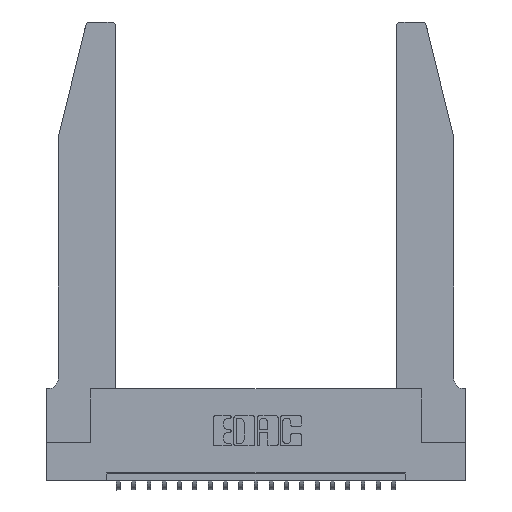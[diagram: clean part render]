
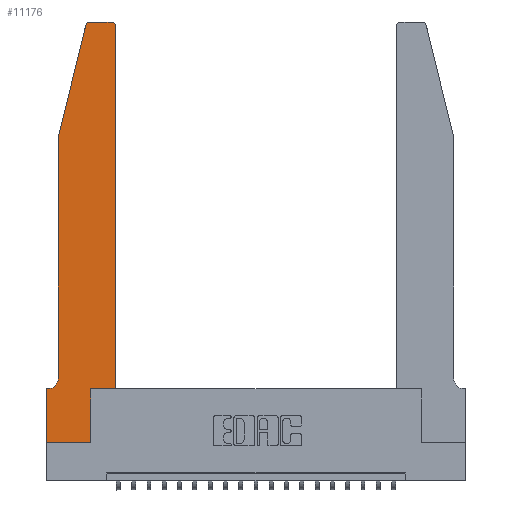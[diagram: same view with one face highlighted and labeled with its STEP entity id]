
A CAD part, top view. The second image highlights one B-rep face of the part: STEP entity #11176.
In plain terms, the highlighted planar face has unit normal (0, 0, 1).
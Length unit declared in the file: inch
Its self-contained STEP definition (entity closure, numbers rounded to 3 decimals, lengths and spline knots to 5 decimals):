
#21 = VERTEX_POINT ( 'NONE', #10559 ) ;
#182 = EDGE_CURVE ( 'NONE', #10941, #19916, #4778, .T. ) ;
#286 = CARTESIAN_POINT ( 'NONE',  ( 0.4505, 0.35, 0.37 ) ) ;
#399 = ORIENTED_EDGE ( 'NONE', *, *, #8018, .T. ) ;
#402 = CARTESIAN_POINT ( 'NONE',  ( 0.0055, 0.42, 0.37 ) ) ;
#699 = DIRECTION ( 'NONE',  ( 0., 0., -1. ) ) ;
#1274 = CARTESIAN_POINT ( 'NONE',  ( 0.4205, 2.75, 0.37 ) ) ;
#1285 = ORIENTED_EDGE ( 'NONE', *, *, #18798, .T. ) ;
#1601 = EDGE_CURVE ( 'NONE', #10240, #8679, #9013, .T. ) ;
#1625 = DIRECTION ( 'NONE',  ( -1., 0., 0. ) ) ;
#1640 = LINE ( 'NONE', #7037, #21762 ) ;
#1647 = VERTEX_POINT ( 'NONE', #5766 ) ;
#2025 = PLANE ( 'NONE',  #16609 ) ;
#2048 = VECTOR ( 'NONE', #10454, 39.37008 ) ;
#2172 = VECTOR ( 'NONE', #3041, 39.37008 ) ;
#2373 = CARTESIAN_POINT ( 'NONE',  ( 0.4205, 2.72, 0.37 ) ) ;
#2537 = VECTOR ( 'NONE', #14966, 39.37008 ) ;
#2605 = VECTOR ( 'NONE', #7820, 39.37008 ) ;
#2988 = CARTESIAN_POINT ( 'NONE',  ( 0.0755, 0.35, 0.37 ) ) ;
#3041 = DIRECTION ( 'NONE',  ( 0., -1., 0. ) ) ;
#3289 = ORIENTED_EDGE ( 'NONE', *, *, #1601, .T. ) ;
#3709 = EDGE_CURVE ( 'NONE', #19916, #10240, #11325, .T. ) ;
#4046 = CARTESIAN_POINT ( 'NONE',  ( 0.4505, 0.35, 0.37 ) ) ;
#4491 = EDGE_CURVE ( 'NONE', #12046, #14449, #1640, .T. ) ;
#4778 = LINE ( 'NONE', #12713, #2605 ) ;
#4792 = DIRECTION ( 'NONE',  ( 1., 0., 0. ) ) ;
#5110 = VECTOR ( 'NONE', #20875, 39.37008 ) ;
#5119 = CARTESIAN_POINT ( 'NONE',  ( 0., 0., 0.37 ) ) ;
#5201 = DIRECTION ( 'NONE',  ( 0., -1., 0. ) ) ;
#5419 = DIRECTION ( 'NONE',  ( 1., 0., 0. ) ) ;
#5566 = DIRECTION ( 'NONE',  ( 0., 0., 1. ) ) ;
#5766 = CARTESIAN_POINT ( 'NONE',  ( 0.2865, 0., 0.37 ) ) ;
#6323 = ORIENTED_EDGE ( 'NONE', *, *, #4491, .T. ) ;
#6458 = EDGE_CURVE ( 'NONE', #18527, #21, #9106, .T. ) ;
#6981 = ORIENTED_EDGE ( 'NONE', *, *, #16920, .T. ) ;
#7037 = CARTESIAN_POINT ( 'NONE',  ( 0.4505, 0.35, 0.37 ) ) ;
#7155 = CARTESIAN_POINT ( 'NONE',  ( 0., 0., 0.37 ) ) ;
#7533 = DIRECTION ( 'NONE',  ( 0., 0., 1. ) ) ;
#7820 = DIRECTION ( 'NONE',  ( -0.239, -0.971, 0. ) ) ;
#8018 = EDGE_CURVE ( 'NONE', #21, #10941, #10651, .T. ) ;
#8276 = CARTESIAN_POINT ( 'NONE',  ( 0.0755, 2., 0.37 ) ) ;
#8469 = CARTESIAN_POINT ( 'NONE',  ( 0.0755, 2., 0.37 ) ) ;
#8679 = VERTEX_POINT ( 'NONE', #9305 ) ;
#9013 = CIRCLE ( 'NONE', #11907, 0.07 ) ;
#9106 = LINE ( 'NONE', #11856, #18732 ) ;
#9305 = CARTESIAN_POINT ( 'NONE',  ( 0.0055, 0.35, 0.37 ) ) ;
#9354 = EDGE_CURVE ( 'NONE', #8679, #9945, #21315, .T. ) ;
#9695 = LINE ( 'NONE', #7155, #5110 ) ;
#9945 = VERTEX_POINT ( 'NONE', #20150 ) ;
#10240 = VERTEX_POINT ( 'NONE', #21269 ) ;
#10300 = CARTESIAN_POINT ( 'NONE',  ( 0.4505, 2.72, 0.37 ) ) ;
#10454 = DIRECTION ( 'NONE',  ( 1., 0., 0. ) ) ;
#10559 = CARTESIAN_POINT ( 'NONE',  ( 0.284, 2.75, 0.37 ) ) ;
#10582 = CIRCLE ( 'NONE', #17485, 0.03 ) ;
#10651 = CIRCLE ( 'NONE', #10993, 0.03 ) ;
#10816 = ORIENTED_EDGE ( 'NONE', *, *, #12298, .T. ) ;
#10941 = VERTEX_POINT ( 'NONE', #20520 ) ;
#10954 = DIRECTION ( 'NONE',  ( 1., 0., 0. ) ) ;
#10993 = AXIS2_PLACEMENT_3D ( 'NONE', #11484, #13179, #4792 ) ;
#11176 = ADVANCED_FACE ( 'NONE', ( #20434 ), #2025, .T. ) ;
#11325 = LINE ( 'NONE', #8469, #2172 ) ;
#11484 = CARTESIAN_POINT ( 'NONE',  ( 0.284, 2.72, 0.37 ) ) ;
#11856 = CARTESIAN_POINT ( 'NONE',  ( 0.2605, 2.75, 0.37 ) ) ;
#11875 = CARTESIAN_POINT ( 'NONE',  ( 0.2865, 0.35, 0.37 ) ) ;
#11907 = AXIS2_PLACEMENT_3D ( 'NONE', #402, #699, #12506 ) ;
#12046 = VERTEX_POINT ( 'NONE', #4046 ) ;
#12298 = EDGE_CURVE ( 'NONE', #18048, #12046, #13878, .T. ) ;
#12506 = DIRECTION ( 'NONE',  ( -1., 0., 0. ) ) ;
#12713 = CARTESIAN_POINT ( 'NONE',  ( 0.0755, 2., 0.37 ) ) ;
#12988 = EDGE_CURVE ( 'NONE', #9945, #13120, #18380, .T. ) ;
#13120 = VERTEX_POINT ( 'NONE', #21273 ) ;
#13179 = DIRECTION ( 'NONE',  ( 0., 0., 1. ) ) ;
#13310 = EDGE_LOOP ( 'NONE', ( #17083, #399, #17147, #17556, #3289, #20088, #13938, #6981, #1285, #10816, #6323, #18278 ) ) ;
#13731 = LINE ( 'NONE', #11875, #20682 ) ;
#13878 = LINE ( 'NONE', #286, #2048 ) ;
#13938 = ORIENTED_EDGE ( 'NONE', *, *, #12988, .T. ) ;
#14449 = VERTEX_POINT ( 'NONE', #10300 ) ;
#14587 = EDGE_CURVE ( 'NONE', #14449, #18527, #10582, .T. ) ;
#14966 = DIRECTION ( 'NONE',  ( -1., 0., 0. ) ) ;
#15383 = CARTESIAN_POINT ( 'NONE',  ( 0.2865, 0.35, 0.37 ) ) ;
#16609 = AXIS2_PLACEMENT_3D ( 'NONE', #19401, #5566, #5419 ) ;
#16920 = EDGE_CURVE ( 'NONE', #13120, #1647, #9695, .T. ) ;
#17083 = ORIENTED_EDGE ( 'NONE', *, *, #6458, .T. ) ;
#17147 = ORIENTED_EDGE ( 'NONE', *, *, #182, .T. ) ;
#17485 = AXIS2_PLACEMENT_3D ( 'NONE', #2373, #7533, #10954 ) ;
#17556 = ORIENTED_EDGE ( 'NONE', *, *, #3709, .T. ) ;
#18048 = VERTEX_POINT ( 'NONE', #15383 ) ;
#18278 = ORIENTED_EDGE ( 'NONE', *, *, #14587, .T. ) ;
#18380 = LINE ( 'NONE', #5119, #19454 ) ;
#18527 = VERTEX_POINT ( 'NONE', #1274 ) ;
#18675 = DIRECTION ( 'NONE',  ( 0., 1., 0. ) ) ;
#18732 = VECTOR ( 'NONE', #1625, 39.37008 ) ;
#18798 = EDGE_CURVE ( 'NONE', #1647, #18048, #13731, .T. ) ;
#19401 = CARTESIAN_POINT ( 'NONE',  ( 0., 0.35, 0.37 ) ) ;
#19454 = VECTOR ( 'NONE', #5201, 39.37008 ) ;
#19916 = VERTEX_POINT ( 'NONE', #8276 ) ;
#20088 = ORIENTED_EDGE ( 'NONE', *, *, #9354, .T. ) ;
#20150 = CARTESIAN_POINT ( 'NONE',  ( 0., 0.35, 0.37 ) ) ;
#20434 = FACE_OUTER_BOUND ( 'NONE', #13310, .T. ) ;
#20520 = CARTESIAN_POINT ( 'NONE',  ( 0.25487, 2.72718, 0.37 ) ) ;
#20682 = VECTOR ( 'NONE', #22045, 39.37008 ) ;
#20875 = DIRECTION ( 'NONE',  ( 1., 0., 0. ) ) ;
#21269 = CARTESIAN_POINT ( 'NONE',  ( 0.0755, 0.42, 0.37 ) ) ;
#21273 = CARTESIAN_POINT ( 'NONE',  ( 0., 0., 0.37 ) ) ;
#21315 = LINE ( 'NONE', #2988, #2537 ) ;
#21762 = VECTOR ( 'NONE', #18675, 39.37008 ) ;
#22045 = DIRECTION ( 'NONE',  ( 0., 1., 0. ) ) ;
